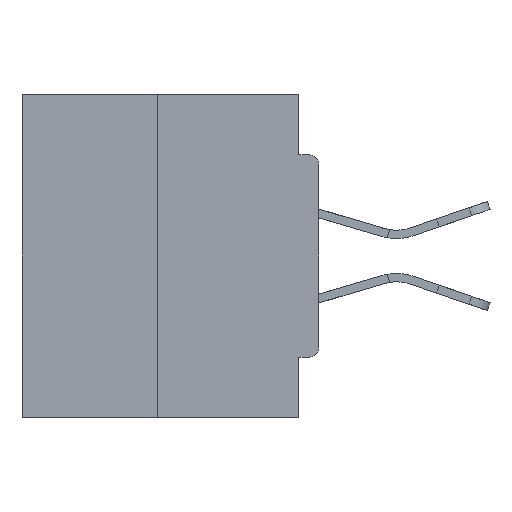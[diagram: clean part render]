
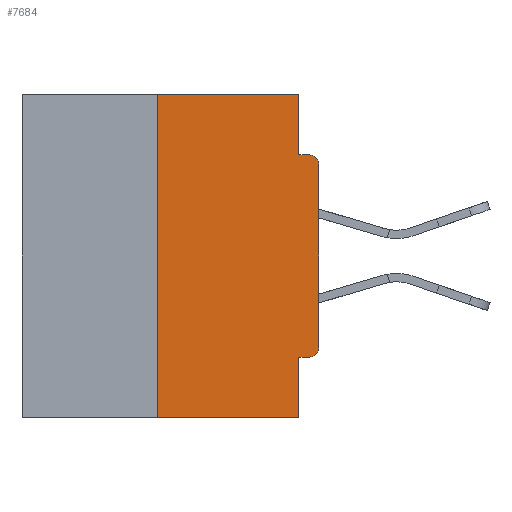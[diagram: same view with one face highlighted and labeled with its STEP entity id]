
A CAD part, left-side view. The second image highlights one B-rep face of the part: STEP entity #7684.
In plain terms, the highlighted planar face has unit normal (-1, 0, 0).
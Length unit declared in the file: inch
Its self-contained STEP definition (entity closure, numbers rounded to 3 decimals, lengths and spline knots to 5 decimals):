
#234 = VECTOR ( 'NONE', #18122, 39.37008 ) ;
#2308 = VERTEX_POINT ( 'NONE', #22597 ) ;
#2410 = ORIENTED_EDGE ( 'NONE', *, *, #34793, .T. ) ;
#3438 = DIRECTION ( 'NONE',  ( 0., 0., 1. ) ) ;
#3583 = VERTEX_POINT ( 'NONE', #25223 ) ;
#4460 = CARTESIAN_POINT ( 'NONE',  ( 0., 0.25, -0.5 ) ) ;
#4712 = CARTESIAN_POINT ( 'NONE',  ( 0., 0.46, 0. ) ) ;
#5143 = DIRECTION ( 'NONE',  ( 0., 0., -1. ) ) ;
#5198 = LINE ( 'NONE', #30004, #25792 ) ;
#5793 = DIRECTION ( 'NONE',  ( 1., 0., 0. ) ) ;
#5874 = ORIENTED_EDGE ( 'NONE', *, *, #31214, .T. ) ;
#5928 = LINE ( 'NONE', #19727, #33702 ) ;
#6175 = CARTESIAN_POINT ( 'NONE',  ( 0., 0.015, -0.1085 ) ) ;
#6334 = VECTOR ( 'NONE', #32675, 39.37008 ) ;
#6344 = CARTESIAN_POINT ( 'NONE',  ( 0., 0.25, 0. ) ) ;
#6712 = CARTESIAN_POINT ( 'NONE',  ( 0., 0., 0. ) ) ;
#7684 = ADVANCED_FACE ( 'NONE', ( #18394 ), #21664, .F. ) ;
#7829 = VERTEX_POINT ( 'NONE', #16521 ) ;
#8148 = DIRECTION ( 'NONE',  ( 0., 0., -1. ) ) ;
#8577 = EDGE_CURVE ( 'NONE', #27846, #22163, #16217, .T. ) ;
#8584 = LINE ( 'NONE', #26379, #234 ) ;
#9431 = DIRECTION ( 'NONE',  ( 0., 0., 1. ) ) ;
#9473 = DIRECTION ( 'NONE',  ( 0., 0., -1. ) ) ;
#10136 = VERTEX_POINT ( 'NONE', #4460 ) ;
#10725 = CARTESIAN_POINT ( 'NONE',  ( 0., 0.015, -0.4065 ) ) ;
#11195 = ORIENTED_EDGE ( 'NONE', *, *, #34302, .T. ) ;
#11744 = LINE ( 'NONE', #18105, #15076 ) ;
#11943 = ORIENTED_EDGE ( 'NONE', *, *, #15691, .F. ) ;
#12023 = CIRCLE ( 'NONE', #15354, 0.015 ) ;
#12118 = EDGE_LOOP ( 'NONE', ( #29213, #21346, #18737, #20532, #33646, #11195, #5874, #2410, #16762, #11943 ) ) ;
#12428 = VERTEX_POINT ( 'NONE', #23674 ) ;
#13796 = CARTESIAN_POINT ( 'NONE',  ( 0., 0.015, -0.3915 ) ) ;
#15076 = VECTOR ( 'NONE', #23532, 39.37008 ) ;
#15107 = EDGE_CURVE ( 'NONE', #27664, #7829, #5928, .T. ) ;
#15354 = AXIS2_PLACEMENT_3D ( 'NONE', #13796, #30077, #19068 ) ;
#15691 = EDGE_CURVE ( 'NONE', #22163, #27664, #11744, .T. ) ;
#15818 = AXIS2_PLACEMENT_3D ( 'NONE', #24484, #5793, #8148 ) ;
#16217 = LINE ( 'NONE', #4712, #29756 ) ;
#16521 = CARTESIAN_POINT ( 'NONE',  ( 0., 0.015, -0.0935 ) ) ;
#16762 = ORIENTED_EDGE ( 'NONE', *, *, #15107, .F. ) ;
#17841 = CARTESIAN_POINT ( 'NONE',  ( 0., 0., -0.1085 ) ) ;
#18105 = CARTESIAN_POINT ( 'NONE',  ( 0., 0.031, 0. ) ) ;
#18122 = DIRECTION ( 'NONE',  ( 0., -1., 0. ) ) ;
#18394 = FACE_OUTER_BOUND ( 'NONE', #12118, .T. ) ;
#18656 = CARTESIAN_POINT ( 'NONE',  ( 0., 0.031, -0.0935 ) ) ;
#18737 = ORIENTED_EDGE ( 'NONE', *, *, #23902, .T. ) ;
#19068 = DIRECTION ( 'NONE',  ( 0., 0., -1. ) ) ;
#19727 = CARTESIAN_POINT ( 'NONE',  ( 0., 0., -0.0935 ) ) ;
#19810 = EDGE_CURVE ( 'NONE', #2308, #12428, #32288, .T. ) ;
#20532 = ORIENTED_EDGE ( 'NONE', *, *, #19810, .F. ) ;
#20799 = AXIS2_PLACEMENT_3D ( 'NONE', #6175, #24997, #9473 ) ;
#21346 = ORIENTED_EDGE ( 'NONE', *, *, #24689, .F. ) ;
#21593 = VERTEX_POINT ( 'NONE', #10725 ) ;
#21664 = PLANE ( 'NONE',  #15818 ) ;
#21777 = CIRCLE ( 'NONE', #20799, 0.015 ) ;
#22163 = VERTEX_POINT ( 'NONE', #26909 ) ;
#22327 = LINE ( 'NONE', #27129, #6334 ) ;
#22597 = CARTESIAN_POINT ( 'NONE',  ( 0., 0.031, -0.4065 ) ) ;
#23532 = DIRECTION ( 'NONE',  ( 0., 0., -1. ) ) ;
#23674 = CARTESIAN_POINT ( 'NONE',  ( 0., 0.031, -0.5 ) ) ;
#23902 = EDGE_CURVE ( 'NONE', #10136, #12428, #8584, .T. ) ;
#24484 = CARTESIAN_POINT ( 'NONE',  ( 0., 0.46, 0. ) ) ;
#24689 = EDGE_CURVE ( 'NONE', #10136, #27846, #5198, .T. ) ;
#24997 = DIRECTION ( 'NONE',  ( -1., 0., 0. ) ) ;
#25173 = DIRECTION ( 'NONE',  ( 0., -1., 0. ) ) ;
#25223 = CARTESIAN_POINT ( 'NONE',  ( 0., 0., -0.3915 ) ) ;
#25741 = DIRECTION ( 'NONE',  ( 0., -1., 0. ) ) ;
#25792 = VECTOR ( 'NONE', #3438, 39.37008 ) ;
#26379 = CARTESIAN_POINT ( 'NONE',  ( 0., 0.46, -0.5 ) ) ;
#26790 = EDGE_CURVE ( 'NONE', #21593, #2308, #22327, .T. ) ;
#26909 = CARTESIAN_POINT ( 'NONE',  ( 0., 0.031, 0. ) ) ;
#27129 = CARTESIAN_POINT ( 'NONE',  ( 0., 0., -0.4065 ) ) ;
#27664 = VERTEX_POINT ( 'NONE', #18656 ) ;
#27846 = VERTEX_POINT ( 'NONE', #6344 ) ;
#28072 = VECTOR ( 'NONE', #5143, 39.37008 ) ;
#28865 = VERTEX_POINT ( 'NONE', #17841 ) ;
#29213 = ORIENTED_EDGE ( 'NONE', *, *, #8577, .F. ) ;
#29756 = VECTOR ( 'NONE', #25741, 39.37008 ) ;
#30004 = CARTESIAN_POINT ( 'NONE',  ( 0., 0.25, 0. ) ) ;
#30077 = DIRECTION ( 'NONE',  ( -1., 0., 0. ) ) ;
#31214 = EDGE_CURVE ( 'NONE', #3583, #28865, #33351, .T. ) ;
#32115 = VECTOR ( 'NONE', #9431, 39.37008 ) ;
#32288 = LINE ( 'NONE', #34749, #28072 ) ;
#32675 = DIRECTION ( 'NONE',  ( 0., 1., 0. ) ) ;
#33351 = LINE ( 'NONE', #6712, #32115 ) ;
#33646 = ORIENTED_EDGE ( 'NONE', *, *, #26790, .F. ) ;
#33702 = VECTOR ( 'NONE', #25173, 39.37008 ) ;
#34302 = EDGE_CURVE ( 'NONE', #21593, #3583, #12023, .T. ) ;
#34749 = CARTESIAN_POINT ( 'NONE',  ( 0., 0.031, -0.5 ) ) ;
#34793 = EDGE_CURVE ( 'NONE', #28865, #7829, #21777, .T. ) ;
